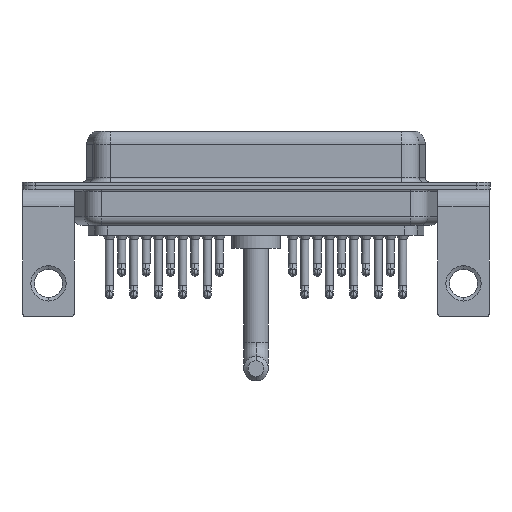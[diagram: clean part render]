
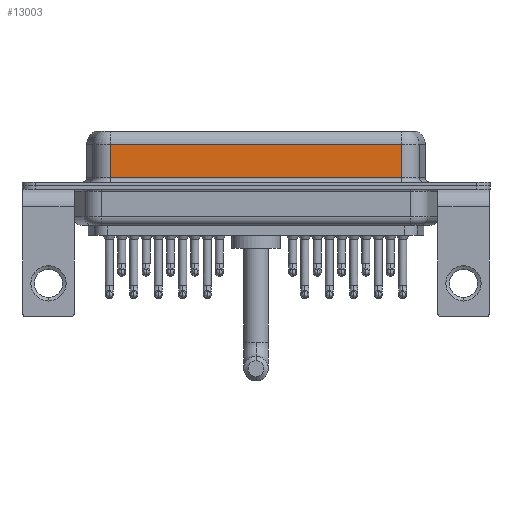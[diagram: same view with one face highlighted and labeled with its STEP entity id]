
A CAD part, front view. The second image highlights one B-rep face of the part: STEP entity #13003.
In plain terms, the highlighted planar face has unit normal (0, -1, 0).
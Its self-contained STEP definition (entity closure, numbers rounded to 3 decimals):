
#371 = CARTESIAN_POINT ( 'NONE',  ( 7.013, -3.95, 4.65 ) ) ;
#860 = VERTEX_POINT ( 'NONE', #18078 ) ;
#1096 = CARTESIAN_POINT ( 'NONE',  ( 40.037, -3.95, 0.9 ) ) ;
#1127 = LINE ( 'NONE', #8364, #11984 ) ;
#1823 = EDGE_CURVE ( 'NONE', #860, #18453, #22526, .T. ) ;
#2740 = VERTEX_POINT ( 'NONE', #3837 ) ;
#3477 = DIRECTION ( 'NONE',  ( 0., 0., 1. ) ) ;
#3837 = CARTESIAN_POINT ( 'NONE',  ( 40.037, -3.95, 4.65 ) ) ;
#4645 = DIRECTION ( 'NONE',  ( 0., 0., -1. ) ) ;
#5816 = EDGE_CURVE ( 'NONE', #2740, #23102, #1127, .T. ) ;
#6310 = DIRECTION ( 'NONE',  ( 1., 0., 0. ) ) ;
#7160 = ORIENTED_EDGE ( 'NONE', *, *, #9496, .F. ) ;
#7958 = ORIENTED_EDGE ( 'NONE', *, *, #5816, .T. ) ;
#8364 = CARTESIAN_POINT ( 'NONE',  ( 40.037, -3.95, 4.65 ) ) ;
#9154 = VECTOR ( 'NONE', #6310, 1000. ) ;
#9496 = EDGE_CURVE ( 'NONE', #2740, #18453, #20882, .T. ) ;
#10463 = CARTESIAN_POINT ( 'NONE',  ( 40.037, -3.95, 6.4 ) ) ;
#11115 = CARTESIAN_POINT ( 'NONE',  ( 40.037, -3.95, 6.4 ) ) ;
#11328 = ORIENTED_EDGE ( 'NONE', *, *, #1823, .T. ) ;
#11984 = VECTOR ( 'NONE', #13825, 1000. ) ;
#12401 = EDGE_LOOP ( 'NONE', ( #7160, #7958, #22106, #11328 ) ) ;
#13003 = ADVANCED_FACE ( 'NONE', ( #19750 ), #21730, .F. ) ;
#13825 = DIRECTION ( 'NONE',  ( -1., 0., 0. ) ) ;
#14092 = LINE ( 'NONE', #19413, #20368 ) ;
#14685 = EDGE_CURVE ( 'NONE', #23102, #860, #14092, .T. ) ;
#15746 = CARTESIAN_POINT ( 'NONE',  ( 40.037, -3.95, 0.9 ) ) ;
#16492 = AXIS2_PLACEMENT_3D ( 'NONE', #11115, #18321, #3477 ) ;
#18078 = CARTESIAN_POINT ( 'NONE',  ( 7.013, -3.95, 0.9 ) ) ;
#18321 = DIRECTION ( 'NONE',  ( 0., 1., 0. ) ) ;
#18453 = VERTEX_POINT ( 'NONE', #15746 ) ;
#19268 = VECTOR ( 'NONE', #4645, 1000. ) ;
#19413 = CARTESIAN_POINT ( 'NONE',  ( 7.013, -3.95, 6.4 ) ) ;
#19750 = FACE_OUTER_BOUND ( 'NONE', #12401, .T. ) ;
#20368 = VECTOR ( 'NONE', #21052, 1000. ) ;
#20882 = LINE ( 'NONE', #10463, #19268 ) ;
#21052 = DIRECTION ( 'NONE',  ( 0., 0., -1. ) ) ;
#21730 = PLANE ( 'NONE',  #16492 ) ;
#22106 = ORIENTED_EDGE ( 'NONE', *, *, #14685, .T. ) ;
#22526 = LINE ( 'NONE', #1096, #9154 ) ;
#23102 = VERTEX_POINT ( 'NONE', #371 ) ;
